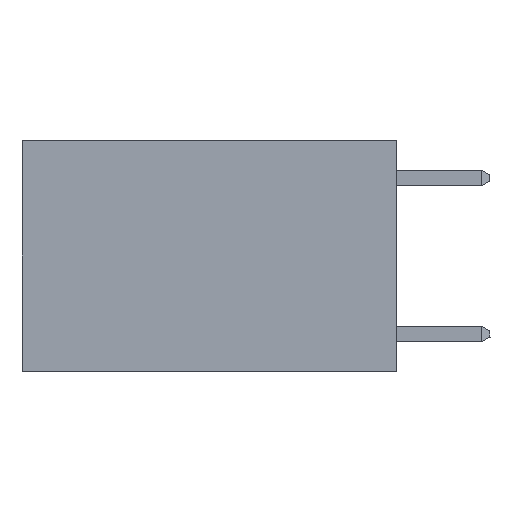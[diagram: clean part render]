
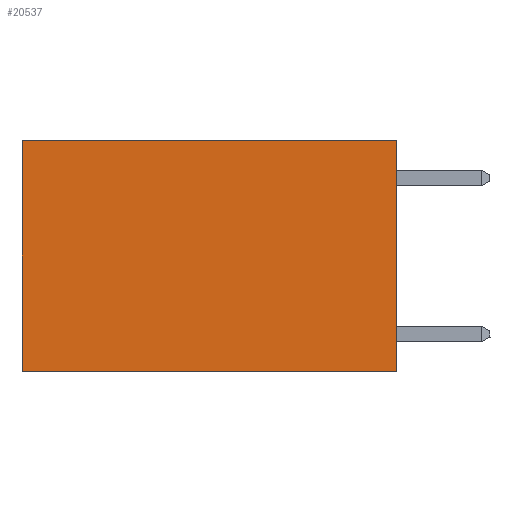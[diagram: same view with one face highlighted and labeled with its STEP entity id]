
A CAD part, left-side view. The second image highlights one B-rep face of the part: STEP entity #20537.
In plain terms, the highlighted planar face has unit normal (-1, 0, 0).
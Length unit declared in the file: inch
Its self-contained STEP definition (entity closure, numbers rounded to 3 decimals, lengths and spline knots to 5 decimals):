
#492 = DIRECTION ( 'NONE',  ( 0., 0., -1. ) ) ;
#909 = EDGE_CURVE ( 'NONE', #5580, #9657, #13339, .T. ) ;
#1608 = FACE_OUTER_BOUND ( 'NONE', #15401, .T. ) ;
#2058 = CARTESIAN_POINT ( 'NONE',  ( 0.2625, 0.6, -0.37 ) ) ;
#3115 = AXIS2_PLACEMENT_3D ( 'NONE', #14720, #3739, #16579 ) ;
#3739 = DIRECTION ( 'NONE',  ( 1., 0., 0. ) ) ;
#3992 = CARTESIAN_POINT ( 'NONE',  ( 0.2625, 0., 0. ) ) ;
#5580 = VERTEX_POINT ( 'NONE', #20049 ) ;
#6269 = CARTESIAN_POINT ( 'NONE',  ( 0.2625, 0.6, 0. ) ) ;
#7371 = ORIENTED_EDGE ( 'NONE', *, *, #16094, .F. ) ;
#8566 = LINE ( 'NONE', #13876, #17779 ) ;
#9460 = LINE ( 'NONE', #11842, #18670 ) ;
#9657 = VERTEX_POINT ( 'NONE', #2058 ) ;
#10224 = DIRECTION ( 'NONE',  ( 0., 0., -1. ) ) ;
#10841 = VECTOR ( 'NONE', #492, 39.37008 ) ;
#11316 = ORIENTED_EDGE ( 'NONE', *, *, #22023, .T. ) ;
#11401 = LINE ( 'NONE', #3992, #10841 ) ;
#11549 = ORIENTED_EDGE ( 'NONE', *, *, #909, .F. ) ;
#11842 = CARTESIAN_POINT ( 'NONE',  ( 0.2625, 0., 0. ) ) ;
#12285 = VERTEX_POINT ( 'NONE', #6269 ) ;
#12824 = PLANE ( 'NONE',  #3115 ) ;
#12947 = CARTESIAN_POINT ( 'NONE',  ( 0.2625, 0., 0. ) ) ;
#13339 = LINE ( 'NONE', #19131, #13388 ) ;
#13388 = VECTOR ( 'NONE', #15538, 39.37008 ) ;
#13747 = DIRECTION ( 'NONE',  ( 0., 1., 0. ) ) ;
#13876 = CARTESIAN_POINT ( 'NONE',  ( 0.2625, 0.6, 0. ) ) ;
#14720 = CARTESIAN_POINT ( 'NONE',  ( 0.2625, 0., 0. ) ) ;
#15315 = VERTEX_POINT ( 'NONE', #12947 ) ;
#15401 = EDGE_LOOP ( 'NONE', ( #18330, #11549, #7371, #11316 ) ) ;
#15538 = DIRECTION ( 'NONE',  ( 0., 1., 0. ) ) ;
#16094 = EDGE_CURVE ( 'NONE', #15315, #5580, #11401, .T. ) ;
#16579 = DIRECTION ( 'NONE',  ( 0., 0., -1. ) ) ;
#17779 = VECTOR ( 'NONE', #10224, 39.37008 ) ;
#18330 = ORIENTED_EDGE ( 'NONE', *, *, #22762, .T. ) ;
#18670 = VECTOR ( 'NONE', #13747, 39.37008 ) ;
#19131 = CARTESIAN_POINT ( 'NONE',  ( 0.2625, 0., -0.37 ) ) ;
#20049 = CARTESIAN_POINT ( 'NONE',  ( 0.2625, 0., -0.37 ) ) ;
#20537 = ADVANCED_FACE ( 'NONE', ( #1608 ), #12824, .F. ) ;
#22023 = EDGE_CURVE ( 'NONE', #15315, #12285, #9460, .T. ) ;
#22762 = EDGE_CURVE ( 'NONE', #12285, #9657, #8566, .T. ) ;
